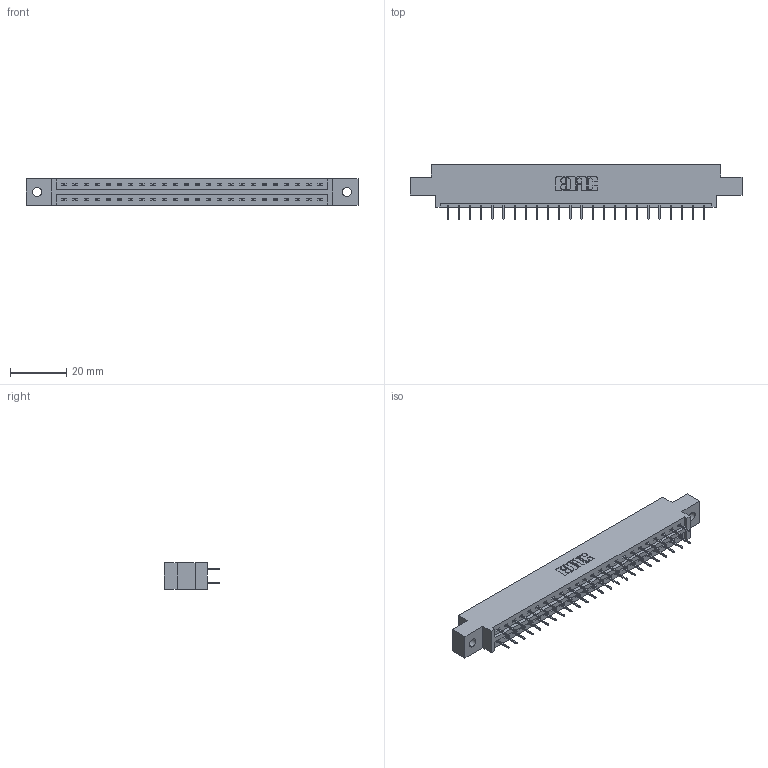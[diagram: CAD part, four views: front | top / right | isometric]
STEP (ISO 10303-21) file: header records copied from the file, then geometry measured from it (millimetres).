
FILE_DESCRIPTION (( 'STEP AP203' ), '1' );
FILE_NAME ('337-048-524-802.STEP', '2018-08-09T09:53:14', ( '' ), ( '' ), 'SwSTEP 2.0', 'SolidWorks 2016', '' );
FILE_SCHEMA (( 'CONFIG_CONTROL_DESIGN' ));
Length unit declared in the file: inch
Products named in the file (3): 337-048-524-802; 337 Part_0.170 Offset - 0.128 Dia; 345-292-001_345-293-124
Assembly tree (49 placements, depth 2):
  337-048-524-802
    337 Part_0.170 Offset - 0.128 Dia
    345-292-001_345-293-124  x48
Bounding box: 118.11 x 19.69 x 9.4 mm (x, y, z)
Volume: 11980.9 mm3; surface area: 12979.8 mm2
Topology: 49 solids, 49 shells, 2902 faces, 8243 edges, 5302 vertices
Faces by surface type: plane 2186, cylinder 716
Entity records: 21145 total; most frequent: CARTESIAN_POINT 3578, ORIENTED_EDGE 3514, DIRECTION 3077, EDGE_CURVE 1757, VECTOR 1633, LINE 1633, VERTEX_POINT 1166, AXIS2_PLACEMENT_3D 722
